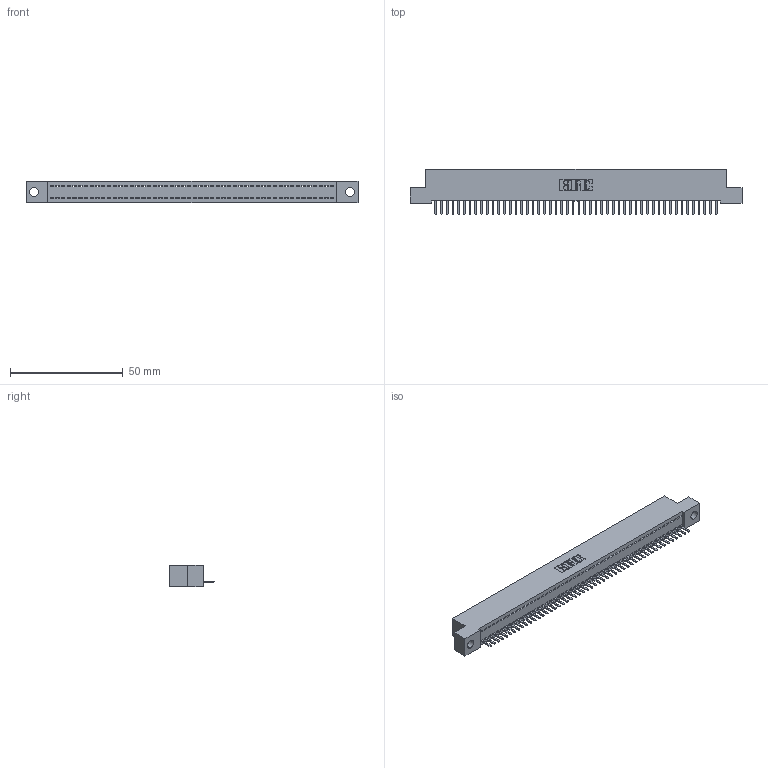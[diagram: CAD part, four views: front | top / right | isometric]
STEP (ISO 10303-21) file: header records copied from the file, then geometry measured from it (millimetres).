
FILE_DESCRIPTION (( 'STEP AP203' ), '1' );
FILE_NAME ('342-050-520-104.STEP', '2018-08-12T19:22:24', ( '' ), ( '' ), 'SwSTEP 2.0', 'SolidWorks 2016', '' );
FILE_SCHEMA (( 'CONFIG_CONTROL_DESIGN' ));
Length unit declared in the file: inch
Products named in the file (3): 342 Part_.156 TH; 345-292-001_345-293-120; 342-050-520-104
Assembly tree (51 placements, depth 2):
  342-050-520-104
    342 Part_.156 TH
    345-292-001_345-293-120  x50
Bounding box: 147.32 x 20.02 x 9.4 mm (x, y, z)
Volume: 12715.6 mm3; surface area: 18180.5 mm2
Topology: 51 solids, 51 shells, 3210 faces, 9499 edges, 6198 vertices
Faces by surface type: plane 2266, cylinder 944
Entity records: 29517 total; most frequent: CARTESIAN_POINT 5108, ORIENTED_EDGE 5082, DIRECTION 4281, EDGE_CURVE 2541, LINE 2409, VECTOR 2409, VERTEX_POINT 1690, AXIS2_PLACEMENT_3D 936
